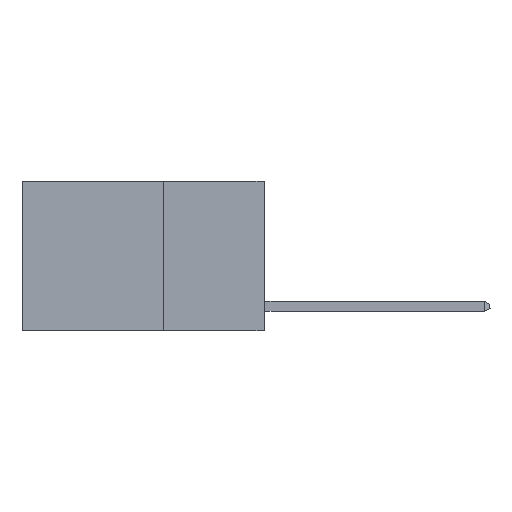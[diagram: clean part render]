
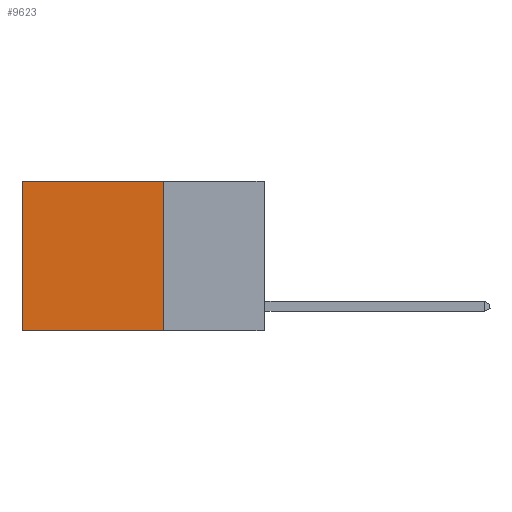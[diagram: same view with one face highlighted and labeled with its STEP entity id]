
A CAD part, left-side view. The second image highlights one B-rep face of the part: STEP entity #9623.
In plain terms, the highlighted planar face has unit normal (-1, 0, 0).
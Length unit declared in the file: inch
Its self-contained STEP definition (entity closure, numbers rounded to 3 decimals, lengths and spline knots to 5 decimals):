
#2492 = VECTOR ( 'NONE', #4377, 39.37008 ) ;
#2749 = CARTESIAN_POINT ( 'NONE',  ( 0.2625, 0.25, 0. ) ) ;
#2896 = CARTESIAN_POINT ( 'NONE',  ( 0.2625, 0.6, 0. ) ) ;
#3291 = DIRECTION ( 'NONE',  ( 0., 1., 0. ) ) ;
#3541 = AXIS2_PLACEMENT_3D ( 'NONE', #12855, #4068, #14336 ) ;
#3696 = CARTESIAN_POINT ( 'NONE',  ( 0.2625, 0.25, -0.37 ) ) ;
#4068 = DIRECTION ( 'NONE',  ( 1., 0., 0. ) ) ;
#4377 = DIRECTION ( 'NONE',  ( 0., 0., -1. ) ) ;
#4924 = VECTOR ( 'NONE', #16620, 39.37008 ) ;
#5142 = EDGE_CURVE ( 'NONE', #9362, #16032, #16627, .T. ) ;
#6905 = VERTEX_POINT ( 'NONE', #14364 ) ;
#6909 = ORIENTED_EDGE ( 'NONE', *, *, #17395, .T. ) ;
#7032 = ORIENTED_EDGE ( 'NONE', *, *, #18859, .F. ) ;
#7163 = FACE_OUTER_BOUND ( 'NONE', #18864, .T. ) ;
#7264 = ORIENTED_EDGE ( 'NONE', *, *, #5142, .F. ) ;
#7744 = VECTOR ( 'NONE', #15981, 39.37008 ) ;
#7895 = ORIENTED_EDGE ( 'NONE', *, *, #15009, .T. ) ;
#9362 = VERTEX_POINT ( 'NONE', #3696 ) ;
#9623 = ADVANCED_FACE ( 'NONE', ( #7163 ), #11258, .F. ) ;
#11258 = PLANE ( 'NONE',  #3541 ) ;
#11558 = VECTOR ( 'NONE', #3291, 39.37008 ) ;
#12089 = CARTESIAN_POINT ( 'NONE',  ( 0.2625, 0.25, 0. ) ) ;
#12194 = CARTESIAN_POINT ( 'NONE',  ( 0.2625, 0.25, 0. ) ) ;
#12855 = CARTESIAN_POINT ( 'NONE',  ( 0.2625, 0.25, 0. ) ) ;
#14204 = LINE ( 'NONE', #2896, #2492 ) ;
#14336 = DIRECTION ( 'NONE',  ( 0., 0., -1. ) ) ;
#14364 = CARTESIAN_POINT ( 'NONE',  ( 0.2625, 0.6, 0. ) ) ;
#15009 = EDGE_CURVE ( 'NONE', #15818, #6905, #15924, .T. ) ;
#15164 = CARTESIAN_POINT ( 'NONE',  ( 0.2625, 0.25, -0.37 ) ) ;
#15818 = VERTEX_POINT ( 'NONE', #12194 ) ;
#15924 = LINE ( 'NONE', #12089, #11558 ) ;
#15981 = DIRECTION ( 'NONE',  ( 0., 0., -1. ) ) ;
#16032 = VERTEX_POINT ( 'NONE', #18605 ) ;
#16620 = DIRECTION ( 'NONE',  ( 0., 1., 0. ) ) ;
#16627 = LINE ( 'NONE', #15164, #4924 ) ;
#17395 = EDGE_CURVE ( 'NONE', #6905, #16032, #14204, .T. ) ;
#18605 = CARTESIAN_POINT ( 'NONE',  ( 0.2625, 0.6, -0.37 ) ) ;
#18859 = EDGE_CURVE ( 'NONE', #15818, #9362, #18995, .T. ) ;
#18864 = EDGE_LOOP ( 'NONE', ( #6909, #7264, #7032, #7895 ) ) ;
#18995 = LINE ( 'NONE', #2749, #7744 ) ;
